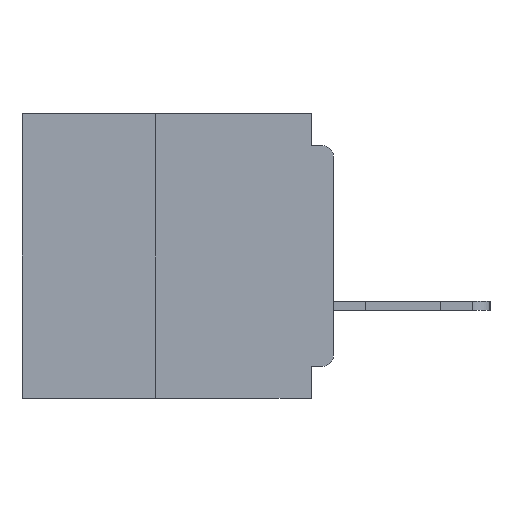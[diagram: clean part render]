
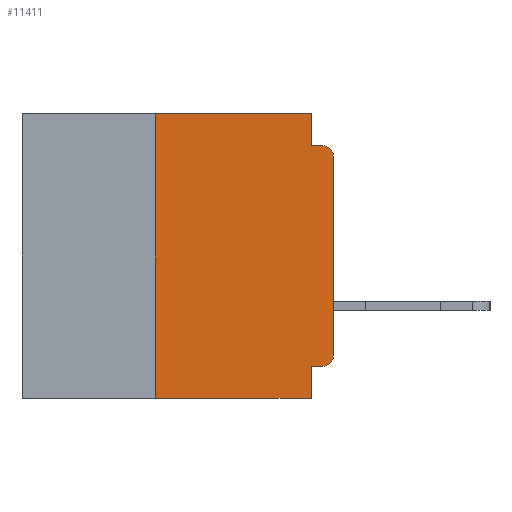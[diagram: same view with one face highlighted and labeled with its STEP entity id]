
A CAD part, left-side view. The second image highlights one B-rep face of the part: STEP entity #11411.
In plain terms, the highlighted planar face has unit normal (-1, 0, 0).
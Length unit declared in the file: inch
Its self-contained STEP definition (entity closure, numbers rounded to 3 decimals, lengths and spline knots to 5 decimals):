
#712 = CARTESIAN_POINT ( 'NONE',  ( 0., 0.015, -0.355 ) ) ;
#1649 = CARTESIAN_POINT ( 'NONE',  ( 0., 0.031, -0.4 ) ) ;
#2161 = CARTESIAN_POINT ( 'NONE',  ( 0., 0.437, 0. ) ) ;
#3418 = ORIENTED_EDGE ( 'NONE', *, *, #15842, .F. ) ;
#3621 = VERTEX_POINT ( 'NONE', #15358 ) ;
#3841 = VERTEX_POINT ( 'NONE', #37665 ) ;
#3992 = CARTESIAN_POINT ( 'NONE',  ( 0., 0.437, 0. ) ) ;
#4011 = VERTEX_POINT ( 'NONE', #5321 ) ;
#5195 = CARTESIAN_POINT ( 'NONE',  ( 0., 0.015, -0.045 ) ) ;
#5321 = CARTESIAN_POINT ( 'NONE',  ( 0., 0.031, 0. ) ) ;
#5410 = LINE ( 'NONE', #1649, #48551 ) ;
#5587 = VERTEX_POINT ( 'NONE', #712 ) ;
#6605 = FACE_OUTER_BOUND ( 'NONE', #31254, .T. ) ;
#7617 = ORIENTED_EDGE ( 'NONE', *, *, #35876, .T. ) ;
#7911 = VECTOR ( 'NONE', #12204, 39.37008 ) ;
#8288 = DIRECTION ( 'NONE',  ( 0., 0., 1. ) ) ;
#9120 = LINE ( 'NONE', #44176, #18847 ) ;
#9666 = EDGE_CURVE ( 'NONE', #5587, #3621, #31590, .T. ) ;
#9982 = VERTEX_POINT ( 'NONE', #42656 ) ;
#10499 = ORIENTED_EDGE ( 'NONE', *, *, #21440, .T. ) ;
#11396 = EDGE_CURVE ( 'NONE', #46932, #9982, #18923, .T. ) ;
#11411 = ADVANCED_FACE ( 'NONE', ( #6605 ), #16189, .F. ) ;
#12204 = DIRECTION ( 'NONE',  ( 0., 0., 1. ) ) ;
#12261 = CARTESIAN_POINT ( 'NONE',  ( 0., 0.031, -0.045 ) ) ;
#14507 = LINE ( 'NONE', #33256, #36777 ) ;
#15358 = CARTESIAN_POINT ( 'NONE',  ( 0., 0.031, -0.355 ) ) ;
#15842 = EDGE_CURVE ( 'NONE', #3621, #48964, #5410, .T. ) ;
#16189 = PLANE ( 'NONE',  #22106 ) ;
#16259 = VECTOR ( 'NONE', #30104, 39.37008 ) ;
#16525 = DIRECTION ( 'NONE',  ( 1., 0., 0. ) ) ;
#18306 = CARTESIAN_POINT ( 'NONE',  ( 0., 0., -0.045 ) ) ;
#18645 = AXIS2_PLACEMENT_3D ( 'NONE', #23555, #52714, #27758 ) ;
#18847 = VECTOR ( 'NONE', #35734, 39.37008 ) ;
#18923 = LINE ( 'NONE', #53758, #7911 ) ;
#19309 = VECTOR ( 'NONE', #26776, 39.37008 ) ;
#19860 = ORIENTED_EDGE ( 'NONE', *, *, #11396, .T. ) ;
#21440 = EDGE_CURVE ( 'NONE', #3841, #48964, #9120, .T. ) ;
#21696 = CARTESIAN_POINT ( 'NONE',  ( 0., 0.031, 0. ) ) ;
#22106 = AXIS2_PLACEMENT_3D ( 'NONE', #3992, #16525, #45824 ) ;
#22667 = EDGE_CURVE ( 'NONE', #48260, #4011, #23992, .T. ) ;
#22902 = AXIS2_PLACEMENT_3D ( 'NONE', #23392, #52530, #27598 ) ;
#23392 = CARTESIAN_POINT ( 'NONE',  ( 0., 0.015, -0.34 ) ) ;
#23555 = CARTESIAN_POINT ( 'NONE',  ( 0., 0.015, -0.06 ) ) ;
#23992 = LINE ( 'NONE', #2161, #43617 ) ;
#26776 = DIRECTION ( 'NONE',  ( 0., -1., 0. ) ) ;
#27598 = DIRECTION ( 'NONE',  ( 0., 0., -1. ) ) ;
#27758 = DIRECTION ( 'NONE',  ( 0., 0., -1. ) ) ;
#28212 = CARTESIAN_POINT ( 'NONE',  ( 0., 0., -0.34 ) ) ;
#29589 = CIRCLE ( 'NONE', #18645, 0.015 ) ;
#29854 = EDGE_CURVE ( 'NONE', #3841, #48260, #14507, .T. ) ;
#30104 = DIRECTION ( 'NONE',  ( 0., 0., -1. ) ) ;
#30196 = ORIENTED_EDGE ( 'NONE', *, *, #22667, .F. ) ;
#31254 = EDGE_LOOP ( 'NONE', ( #19860, #45748, #31951, #43411, #30196, #47442, #10499, #3418, #34914, #7617 ) ) ;
#31590 = LINE ( 'NONE', #39779, #53739 ) ;
#31760 = LINE ( 'NONE', #18306, #19309 ) ;
#31951 = ORIENTED_EDGE ( 'NONE', *, *, #43260, .F. ) ;
#32683 = EDGE_CURVE ( 'NONE', #4011, #42356, #49637, .T. ) ;
#32814 = CARTESIAN_POINT ( 'NONE',  ( 0., 0.25, 0. ) ) ;
#33256 = CARTESIAN_POINT ( 'NONE',  ( 0., 0.25, -0.4 ) ) ;
#34914 = ORIENTED_EDGE ( 'NONE', *, *, #9666, .F. ) ;
#35734 = DIRECTION ( 'NONE',  ( 0., -1., 0. ) ) ;
#35876 = EDGE_CURVE ( 'NONE', #5587, #46932, #45992, .T. ) ;
#36777 = VECTOR ( 'NONE', #8288, 39.37008 ) ;
#37665 = CARTESIAN_POINT ( 'NONE',  ( 0., 0.25, -0.4 ) ) ;
#39375 = DIRECTION ( 'NONE',  ( 0., 0., -1. ) ) ;
#39779 = CARTESIAN_POINT ( 'NONE',  ( 0., 0., -0.355 ) ) ;
#42356 = VERTEX_POINT ( 'NONE', #12261 ) ;
#42656 = CARTESIAN_POINT ( 'NONE',  ( 0., 0., -0.06 ) ) ;
#43260 = EDGE_CURVE ( 'NONE', #42356, #49611, #31760, .T. ) ;
#43411 = ORIENTED_EDGE ( 'NONE', *, *, #32683, .F. ) ;
#43617 = VECTOR ( 'NONE', #43876, 39.37008 ) ;
#43876 = DIRECTION ( 'NONE',  ( 0., -1., 0. ) ) ;
#44176 = CARTESIAN_POINT ( 'NONE',  ( 0., 0.437, -0.4 ) ) ;
#45748 = ORIENTED_EDGE ( 'NONE', *, *, #52593, .T. ) ;
#45824 = DIRECTION ( 'NONE',  ( 0., 0., -1. ) ) ;
#45908 = CARTESIAN_POINT ( 'NONE',  ( 0., 0.031, -0.4 ) ) ;
#45992 = CIRCLE ( 'NONE', #22902, 0.015 ) ;
#46932 = VERTEX_POINT ( 'NONE', #28212 ) ;
#47442 = ORIENTED_EDGE ( 'NONE', *, *, #29854, .F. ) ;
#48260 = VERTEX_POINT ( 'NONE', #32814 ) ;
#48551 = VECTOR ( 'NONE', #39375, 39.37008 ) ;
#48964 = VERTEX_POINT ( 'NONE', #45908 ) ;
#49611 = VERTEX_POINT ( 'NONE', #5195 ) ;
#49637 = LINE ( 'NONE', #21696, #16259 ) ;
#52078 = DIRECTION ( 'NONE',  ( 0., 1., 0. ) ) ;
#52530 = DIRECTION ( 'NONE',  ( -1., 0., 0. ) ) ;
#52593 = EDGE_CURVE ( 'NONE', #9982, #49611, #29589, .T. ) ;
#52714 = DIRECTION ( 'NONE',  ( -1., 0., 0. ) ) ;
#53739 = VECTOR ( 'NONE', #52078, 39.37008 ) ;
#53758 = CARTESIAN_POINT ( 'NONE',  ( 0., 0., 0. ) ) ;
